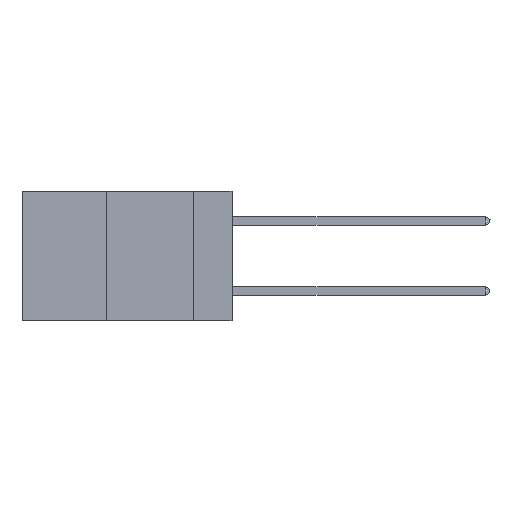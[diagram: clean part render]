
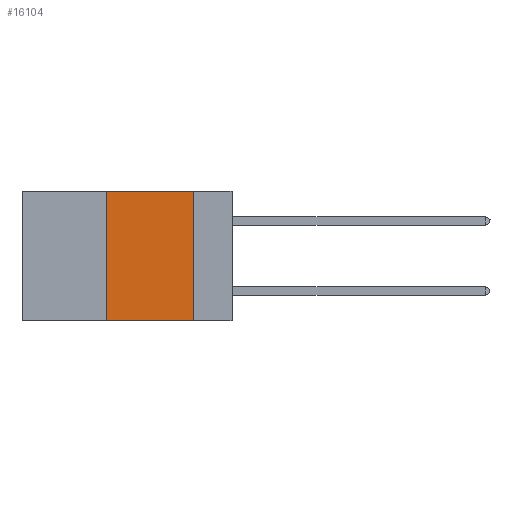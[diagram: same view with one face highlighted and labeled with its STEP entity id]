
A CAD part, left-side view. The second image highlights one B-rep face of the part: STEP entity #16104.
In plain terms, the highlighted planar face has unit normal (-1, 0, 0).
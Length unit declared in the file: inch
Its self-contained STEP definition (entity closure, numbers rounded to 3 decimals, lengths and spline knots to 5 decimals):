
#427 = DIRECTION ( 'NONE',  ( 0., -1., 0. ) ) ;
#615 = DIRECTION ( 'NONE',  ( 0., 0., 1. ) ) ;
#1221 = VECTOR ( 'NONE', #10582, 39.37008 ) ;
#1872 = VECTOR ( 'NONE', #615, 39.37008 ) ;
#2059 = CARTESIAN_POINT ( 'NONE',  ( 0., 0.11, -0.37 ) ) ;
#2841 = VERTEX_POINT ( 'NONE', #11369 ) ;
#3240 = CARTESIAN_POINT ( 'NONE',  ( 0., 0.11, 0. ) ) ;
#3333 = VECTOR ( 'NONE', #3502, 39.37008 ) ;
#3502 = DIRECTION ( 'NONE',  ( 0., 0., -1. ) ) ;
#3618 = EDGE_CURVE ( 'NONE', #19093, #5916, #20675, .T. ) ;
#4021 = DIRECTION ( 'NONE',  ( 1., 0., 0. ) ) ;
#4132 = ORIENTED_EDGE ( 'NONE', *, *, #24925, .F. ) ;
#4447 = ORIENTED_EDGE ( 'NONE', *, *, #25191, .T. ) ;
#5916 = VERTEX_POINT ( 'NONE', #9516 ) ;
#6449 = LINE ( 'NONE', #16593, #22671 ) ;
#9516 = CARTESIAN_POINT ( 'NONE',  ( 0., 0.36, 0. ) ) ;
#9849 = EDGE_CURVE ( 'NONE', #5916, #2841, #6449, .T. ) ;
#10582 = DIRECTION ( 'NONE',  ( 0., -1., 0. ) ) ;
#11369 = CARTESIAN_POINT ( 'NONE',  ( 0., 0.11, 0. ) ) ;
#11958 = EDGE_LOOP ( 'NONE', ( #4132, #13707, #19677, #4447 ) ) ;
#13707 = ORIENTED_EDGE ( 'NONE', *, *, #9849, .F. ) ;
#14186 = PLANE ( 'NONE',  #18325 ) ;
#14783 = CARTESIAN_POINT ( 'NONE',  ( 0., 0.36, 0. ) ) ;
#15171 = CARTESIAN_POINT ( 'NONE',  ( 0., 0.36, -0.37 ) ) ;
#16104 = ADVANCED_FACE ( 'NONE', ( #22577 ), #14186, .F. ) ;
#16300 = DIRECTION ( 'NONE',  ( 0., 0., -1. ) ) ;
#16593 = CARTESIAN_POINT ( 'NONE',  ( 0., 0.6, 0. ) ) ;
#18325 = AXIS2_PLACEMENT_3D ( 'NONE', #24595, #4021, #16300 ) ;
#19093 = VERTEX_POINT ( 'NONE', #15171 ) ;
#19677 = ORIENTED_EDGE ( 'NONE', *, *, #3618, .F. ) ;
#20675 = LINE ( 'NONE', #14783, #1872 ) ;
#20861 = LINE ( 'NONE', #25021, #1221 ) ;
#22577 = FACE_OUTER_BOUND ( 'NONE', #11958, .T. ) ;
#22671 = VECTOR ( 'NONE', #427, 39.37008 ) ;
#23293 = VERTEX_POINT ( 'NONE', #2059 ) ;
#24595 = CARTESIAN_POINT ( 'NONE',  ( 0., 0.6, 0. ) ) ;
#24925 = EDGE_CURVE ( 'NONE', #2841, #23293, #25954, .T. ) ;
#25021 = CARTESIAN_POINT ( 'NONE',  ( 0., 0.6, -0.37 ) ) ;
#25191 = EDGE_CURVE ( 'NONE', #19093, #23293, #20861, .T. ) ;
#25954 = LINE ( 'NONE', #3240, #3333 ) ;
